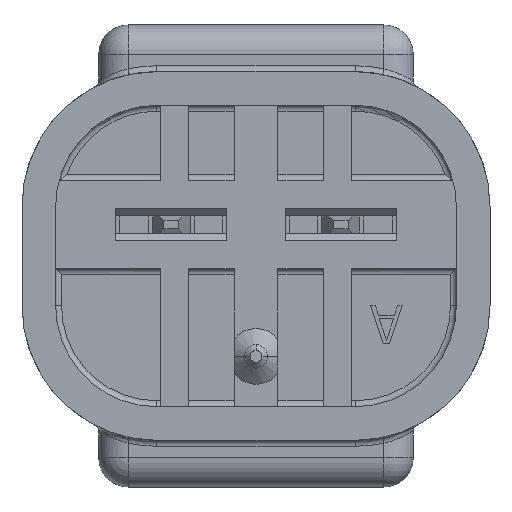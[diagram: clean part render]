
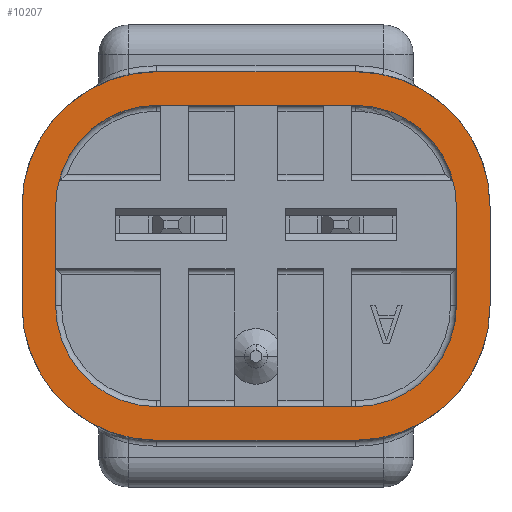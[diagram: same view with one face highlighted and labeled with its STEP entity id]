
A CAD part, front view. The second image highlights one B-rep face of the part: STEP entity #10207.
In plain terms, the highlighted planar face has unit normal (0, -1, 0).
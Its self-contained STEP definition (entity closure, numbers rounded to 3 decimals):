
#104 = VECTOR ( 'NONE', #8929, 1000. ) ;
#213 = ORIENTED_EDGE ( 'NONE', *, *, #11247, .F. ) ;
#219 = CIRCLE ( 'NONE', #7426, 3.45 ) ;
#226 = ORIENTED_EDGE ( 'NONE', *, *, #2216, .T. ) ;
#308 = DIRECTION ( 'NONE',  ( 0., 0., 1. ) ) ;
#351 = CARTESIAN_POINT ( 'NONE',  ( -6.85, -5.75, -1.7 ) ) ;
#364 = DIRECTION ( 'NONE',  ( -1., 0., 0. ) ) ;
#365 = EDGE_CURVE ( 'NONE', #2789, #2506, #4581, .T. ) ;
#525 = ORIENTED_EDGE ( 'NONE', *, *, #8699, .T. ) ;
#578 = ORIENTED_EDGE ( 'NONE', *, *, #1042, .F. ) ;
#626 = CARTESIAN_POINT ( 'NONE',  ( 3.4, -5.75, 1.7 ) ) ;
#671 = EDGE_LOOP ( 'NONE', ( #12040, #7450, #10533, #11657, #3069, #213, #8268, #578 ) ) ;
#732 = LINE ( 'NONE', #5906, #7206 ) ;
#845 = CARTESIAN_POINT ( 'NONE',  ( 6.85, -5.75, 1.7 ) ) ;
#1042 = EDGE_CURVE ( 'NONE', #7910, #4226, #3623, .T. ) ;
#1172 = CARTESIAN_POINT ( 'NONE',  ( 3.4, -5.75, -5.15 ) ) ;
#1185 = LINE ( 'NONE', #7001, #104 ) ;
#1345 = CARTESIAN_POINT ( 'NONE',  ( 6.85, -5.75, 1.7 ) ) ;
#1383 = ORIENTED_EDGE ( 'NONE', *, *, #7530, .T. ) ;
#1545 = AXIS2_PLACEMENT_3D ( 'NONE', #3372, #7289, #2404 ) ;
#1570 = CARTESIAN_POINT ( 'NONE',  ( 8., -5.75, 1.7 ) ) ;
#1688 = EDGE_CURVE ( 'NONE', #5841, #7107, #219, .T. ) ;
#1768 = DIRECTION ( 'NONE',  ( 0., 1., 0. ) ) ;
#1959 = CARTESIAN_POINT ( 'NONE',  ( 3.4, -5.75, 5.15 ) ) ;
#2161 = DIRECTION ( 'NONE',  ( -1., 0., 0. ) ) ;
#2216 = EDGE_CURVE ( 'NONE', #2789, #9950, #1185, .T. ) ;
#2353 = DIRECTION ( 'NONE',  ( -1., 0., 0. ) ) ;
#2404 = DIRECTION ( 'NONE',  ( 0., 0., 1. ) ) ;
#2439 = CARTESIAN_POINT ( 'NONE',  ( 8., -5.75, -1.7 ) ) ;
#2506 = VERTEX_POINT ( 'NONE', #2995 ) ;
#2736 = DIRECTION ( 'NONE',  ( 0., -1., 0. ) ) ;
#2745 = EDGE_CURVE ( 'NONE', #9443, #10400, #7252, .T. ) ;
#2789 = VERTEX_POINT ( 'NONE', #351 ) ;
#2816 = EDGE_LOOP ( 'NONE', ( #4239, #525, #10267, #226, #9563, #1383, #3340, #5456 ) ) ;
#2941 = DIRECTION ( 'NONE',  ( 0., 0., -1. ) ) ;
#2995 = CARTESIAN_POINT ( 'NONE',  ( -3.4, -5.75, -5.15 ) ) ;
#3067 = AXIS2_PLACEMENT_3D ( 'NONE', #8046, #11145, #6242 ) ;
#3069 = ORIENTED_EDGE ( 'NONE', *, *, #3273, .F. ) ;
#3273 = EDGE_CURVE ( 'NONE', #4346, #7324, #10193, .T. ) ;
#3340 = ORIENTED_EDGE ( 'NONE', *, *, #1688, .T. ) ;
#3372 = CARTESIAN_POINT ( 'NONE',  ( 3.4, -5.75, 1.7 ) ) ;
#3388 = DIRECTION ( 'NONE',  ( 0., 1., 0. ) ) ;
#3623 = CIRCLE ( 'NONE', #8559, 4.6 ) ;
#3811 = DIRECTION ( 'NONE',  ( 1., 0., 0. ) ) ;
#4014 = VERTEX_POINT ( 'NONE', #6170 ) ;
#4180 = DIRECTION ( 'NONE',  ( 0., -1., 0. ) ) ;
#4226 = VERTEX_POINT ( 'NONE', #6311 ) ;
#4239 = ORIENTED_EDGE ( 'NONE', *, *, #9700, .F. ) ;
#4346 = VERTEX_POINT ( 'NONE', #9777 ) ;
#4386 = CARTESIAN_POINT ( 'NONE',  ( 3.4, -5.75, -5.15 ) ) ;
#4501 = VECTOR ( 'NONE', #308, 1000. ) ;
#4504 = CIRCLE ( 'NONE', #11316, 4.6 ) ;
#4581 = CIRCLE ( 'NONE', #6236, 3.45 ) ;
#4649 = CARTESIAN_POINT ( 'NONE',  ( -3.4, -5.75, -6.3 ) ) ;
#4719 = CARTESIAN_POINT ( 'NONE',  ( 6.85, -5.75, -1.7 ) ) ;
#4929 = DIRECTION ( 'NONE',  ( 1., 0., 0. ) ) ;
#5155 = CARTESIAN_POINT ( 'NONE',  ( -3.4, -5.75, -1.7 ) ) ;
#5217 = LINE ( 'NONE', #9143, #4501 ) ;
#5293 = EDGE_CURVE ( 'NONE', #7324, #9443, #9158, .T. ) ;
#5456 = ORIENTED_EDGE ( 'NONE', *, *, #9091, .T. ) ;
#5466 = CARTESIAN_POINT ( 'NONE',  ( 3.4, -5.75, 6.3 ) ) ;
#5742 = CARTESIAN_POINT ( 'NONE',  ( -3.4, -5.75, 6.3 ) ) ;
#5745 = AXIS2_PLACEMENT_3D ( 'NONE', #7632, #1768, #9510 ) ;
#5841 = VERTEX_POINT ( 'NONE', #1959 ) ;
#5906 = CARTESIAN_POINT ( 'NONE',  ( -3.4, -5.75, 5.15 ) ) ;
#5973 = DIRECTION ( 'NONE',  ( 0., 1., 0. ) ) ;
#6170 = CARTESIAN_POINT ( 'NONE',  ( 3.4, -5.75, -6.3 ) ) ;
#6236 = AXIS2_PLACEMENT_3D ( 'NONE', #5155, #4180, #364 ) ;
#6242 = DIRECTION ( 'NONE',  ( 1., 0., 0. ) ) ;
#6254 = VECTOR ( 'NONE', #3811, 1000. ) ;
#6311 = CARTESIAN_POINT ( 'NONE',  ( -8., -5.75, -1.7 ) ) ;
#6357 = EDGE_CURVE ( 'NONE', #4014, #7910, #7970, .T. ) ;
#6508 = EDGE_CURVE ( 'NONE', #9950, #9162, #11957, .T. ) ;
#6947 = VERTEX_POINT ( 'NONE', #4386 ) ;
#7001 = CARTESIAN_POINT ( 'NONE',  ( -6.85, -5.75, -1.7 ) ) ;
#7107 = VERTEX_POINT ( 'NONE', #845 ) ;
#7200 = FACE_BOUND ( 'NONE', #2816, .T. ) ;
#7206 = VECTOR ( 'NONE', #4929, 1000. ) ;
#7252 = LINE ( 'NONE', #1570, #9160 ) ;
#7289 = DIRECTION ( 'NONE',  ( 0., 1., 0. ) ) ;
#7324 = VERTEX_POINT ( 'NONE', #5466 ) ;
#7426 = AXIS2_PLACEMENT_3D ( 'NONE', #626, #8758, #7782 ) ;
#7450 = ORIENTED_EDGE ( 'NONE', *, *, #11134, .F. ) ;
#7466 = CARTESIAN_POINT ( 'NONE',  ( -6.85, -5.75, 1.7 ) ) ;
#7530 = EDGE_CURVE ( 'NONE', #9162, #5841, #732, .T. ) ;
#7632 = CARTESIAN_POINT ( 'NONE',  ( -3.4, -5.75, 1.7 ) ) ;
#7782 = DIRECTION ( 'NONE',  ( 0., 0., 1. ) ) ;
#7806 = AXIS2_PLACEMENT_3D ( 'NONE', #11569, #2736, #12602 ) ;
#7910 = VERTEX_POINT ( 'NONE', #4649 ) ;
#7970 = LINE ( 'NONE', #11128, #9239 ) ;
#7980 = FACE_OUTER_BOUND ( 'NONE', #671, .T. ) ;
#8046 = CARTESIAN_POINT ( 'NONE',  ( 0., -5.75, 0. ) ) ;
#8132 = DIRECTION ( 'NONE',  ( -1., 0., 0. ) ) ;
#8268 = ORIENTED_EDGE ( 'NONE', *, *, #9184, .F. ) ;
#8316 = CARTESIAN_POINT ( 'NONE',  ( 3.4, -5.75, -1.7 ) ) ;
#8559 = AXIS2_PLACEMENT_3D ( 'NONE', #11895, #5973, #2941 ) ;
#8699 = EDGE_CURVE ( 'NONE', #6947, #2506, #10974, .T. ) ;
#8758 = DIRECTION ( 'NONE',  ( 0., 1., 0. ) ) ;
#8929 = DIRECTION ( 'NONE',  ( 0., 0., 1. ) ) ;
#9017 = CARTESIAN_POINT ( 'NONE',  ( -3.4, -5.75, 5.15 ) ) ;
#9030 = AXIS2_PLACEMENT_3D ( 'NONE', #9313, #3388, #2353 ) ;
#9091 = EDGE_CURVE ( 'NONE', #7107, #12210, #11159, .T. ) ;
#9143 = CARTESIAN_POINT ( 'NONE',  ( -8., -5.75, -1.7 ) ) ;
#9158 = CIRCLE ( 'NONE', #1545, 4.6 ) ;
#9160 = VECTOR ( 'NONE', #11000, 1000. ) ;
#9162 = VERTEX_POINT ( 'NONE', #9017 ) ;
#9184 = EDGE_CURVE ( 'NONE', #4226, #12614, #5217, .T. ) ;
#9214 = DIRECTION ( 'NONE',  ( 0., 0., -1. ) ) ;
#9239 = VECTOR ( 'NONE', #2161, 1000. ) ;
#9255 = CIRCLE ( 'NONE', #7806, 3.45 ) ;
#9313 = CARTESIAN_POINT ( 'NONE',  ( -3.4, -5.75, 1.7 ) ) ;
#9344 = DIRECTION ( 'NONE',  ( 0., 1., 0. ) ) ;
#9406 = DIRECTION ( 'NONE',  ( 1., 0., 0. ) ) ;
#9443 = VERTEX_POINT ( 'NONE', #12106 ) ;
#9510 = DIRECTION ( 'NONE',  ( -1., 0., 0. ) ) ;
#9563 = ORIENTED_EDGE ( 'NONE', *, *, #6508, .T. ) ;
#9607 = VECTOR ( 'NONE', #9214, 1000. ) ;
#9700 = EDGE_CURVE ( 'NONE', #6947, #12210, #9255, .T. ) ;
#9777 = CARTESIAN_POINT ( 'NONE',  ( -3.4, -5.75, 6.3 ) ) ;
#9950 = VERTEX_POINT ( 'NONE', #7466 ) ;
#10008 = VECTOR ( 'NONE', #8132, 1000. ) ;
#10193 = LINE ( 'NONE', #5742, #6254 ) ;
#10207 = ADVANCED_FACE ( 'NONE', ( #7200, #7980 ), #12041, .F. ) ;
#10267 = ORIENTED_EDGE ( 'NONE', *, *, #365, .F. ) ;
#10400 = VERTEX_POINT ( 'NONE', #2439 ) ;
#10533 = ORIENTED_EDGE ( 'NONE', *, *, #2745, .F. ) ;
#10974 = LINE ( 'NONE', #1172, #10008 ) ;
#11000 = DIRECTION ( 'NONE',  ( 0., 0., -1. ) ) ;
#11100 = CIRCLE ( 'NONE', #9030, 4.6 ) ;
#11128 = CARTESIAN_POINT ( 'NONE',  ( 3.4, -5.75, -6.3 ) ) ;
#11134 = EDGE_CURVE ( 'NONE', #10400, #4014, #4504, .T. ) ;
#11145 = DIRECTION ( 'NONE',  ( 0., 1., 0. ) ) ;
#11159 = LINE ( 'NONE', #1345, #9607 ) ;
#11247 = EDGE_CURVE ( 'NONE', #12614, #4346, #11100, .T. ) ;
#11316 = AXIS2_PLACEMENT_3D ( 'NONE', #8316, #9344, #9406 ) ;
#11569 = CARTESIAN_POINT ( 'NONE',  ( 3.4, -5.75, -1.7 ) ) ;
#11657 = ORIENTED_EDGE ( 'NONE', *, *, #5293, .F. ) ;
#11895 = CARTESIAN_POINT ( 'NONE',  ( -3.4, -5.75, -1.7 ) ) ;
#11957 = CIRCLE ( 'NONE', #5745, 3.45 ) ;
#12040 = ORIENTED_EDGE ( 'NONE', *, *, #6357, .F. ) ;
#12041 = PLANE ( 'NONE',  #3067 ) ;
#12106 = CARTESIAN_POINT ( 'NONE',  ( 8., -5.75, 1.7 ) ) ;
#12210 = VERTEX_POINT ( 'NONE', #4719 ) ;
#12467 = CARTESIAN_POINT ( 'NONE',  ( -8., -5.75, 1.7 ) ) ;
#12602 = DIRECTION ( 'NONE',  ( 0., 0., -1. ) ) ;
#12614 = VERTEX_POINT ( 'NONE', #12467 ) ;
